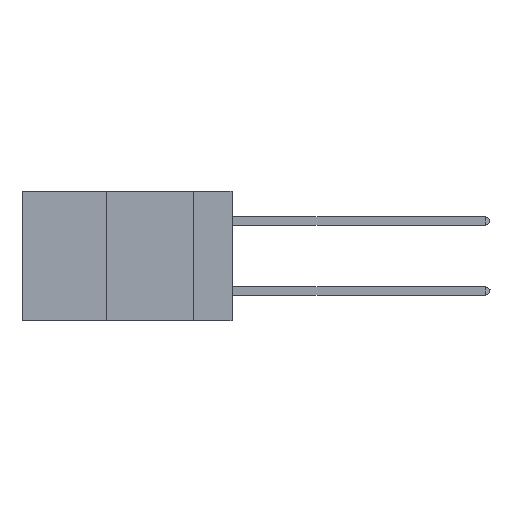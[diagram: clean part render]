
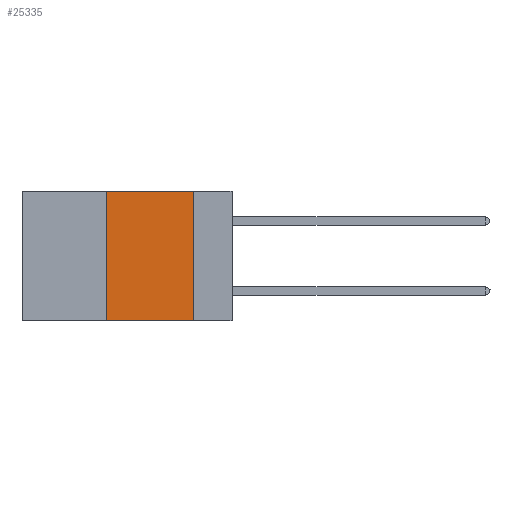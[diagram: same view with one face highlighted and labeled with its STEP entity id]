
A CAD part, left-side view. The second image highlights one B-rep face of the part: STEP entity #25335.
In plain terms, the highlighted planar face has unit normal (-1, 0, 0).
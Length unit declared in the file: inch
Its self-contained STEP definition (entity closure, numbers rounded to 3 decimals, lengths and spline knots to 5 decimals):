
#167 = ORIENTED_EDGE ( 'NONE', *, *, #28785, .F. ) ;
#292 = DIRECTION ( 'NONE',  ( 0., 0., 1. ) ) ;
#1454 = ORIENTED_EDGE ( 'NONE', *, *, #9714, .F. ) ;
#2374 = CARTESIAN_POINT ( 'NONE',  ( 0., 0.36, 0. ) ) ;
#2908 = CARTESIAN_POINT ( 'NONE',  ( 0., 0.11, 0. ) ) ;
#3397 = DIRECTION ( 'NONE',  ( 0., 0., -1. ) ) ;
#7265 = VECTOR ( 'NONE', #292, 39.37008 ) ;
#8159 = LINE ( 'NONE', #2908, #12400 ) ;
#9714 = EDGE_CURVE ( 'NONE', #14563, #24403, #8159, .T. ) ;
#9839 = EDGE_CURVE ( 'NONE', #25215, #24403, #22517, .T. ) ;
#10575 = ORIENTED_EDGE ( 'NONE', *, *, #9839, .T. ) ;
#12022 = EDGE_CURVE ( 'NONE', #18421, #14563, #22094, .T. ) ;
#12042 = VECTOR ( 'NONE', #26512, 39.37008 ) ;
#12400 = VECTOR ( 'NONE', #21106, 39.37008 ) ;
#14563 = VERTEX_POINT ( 'NONE', #26400 ) ;
#15350 = CARTESIAN_POINT ( 'NONE',  ( 0., 0.6, -0.37 ) ) ;
#16027 = CARTESIAN_POINT ( 'NONE',  ( 0., 0.6, 0. ) ) ;
#16731 = LINE ( 'NONE', #2374, #7265 ) ;
#17339 = AXIS2_PLACEMENT_3D ( 'NONE', #25826, #23174, #3397 ) ;
#17913 = DIRECTION ( 'NONE',  ( 0., -1., 0. ) ) ;
#18421 = VERTEX_POINT ( 'NONE', #21714 ) ;
#19983 = VECTOR ( 'NONE', #17913, 39.37008 ) ;
#21106 = DIRECTION ( 'NONE',  ( 0., 0., -1. ) ) ;
#21714 = CARTESIAN_POINT ( 'NONE',  ( 0., 0.36, 0. ) ) ;
#21986 = CARTESIAN_POINT ( 'NONE',  ( 0., 0.11, -0.37 ) ) ;
#22094 = LINE ( 'NONE', #16027, #19983 ) ;
#22517 = LINE ( 'NONE', #15350, #12042 ) ;
#23174 = DIRECTION ( 'NONE',  ( 1., 0., 0. ) ) ;
#24403 = VERTEX_POINT ( 'NONE', #21986 ) ;
#25215 = VERTEX_POINT ( 'NONE', #25732 ) ;
#25277 = EDGE_LOOP ( 'NONE', ( #1454, #27026, #167, #10575 ) ) ;
#25335 = ADVANCED_FACE ( 'NONE', ( #29018 ), #28104, .F. ) ;
#25732 = CARTESIAN_POINT ( 'NONE',  ( 0., 0.36, -0.37 ) ) ;
#25826 = CARTESIAN_POINT ( 'NONE',  ( 0., 0.6, 0. ) ) ;
#26400 = CARTESIAN_POINT ( 'NONE',  ( 0., 0.11, 0. ) ) ;
#26512 = DIRECTION ( 'NONE',  ( 0., -1., 0. ) ) ;
#27026 = ORIENTED_EDGE ( 'NONE', *, *, #12022, .F. ) ;
#28104 = PLANE ( 'NONE',  #17339 ) ;
#28785 = EDGE_CURVE ( 'NONE', #25215, #18421, #16731, .T. ) ;
#29018 = FACE_OUTER_BOUND ( 'NONE', #25277, .T. ) ;
